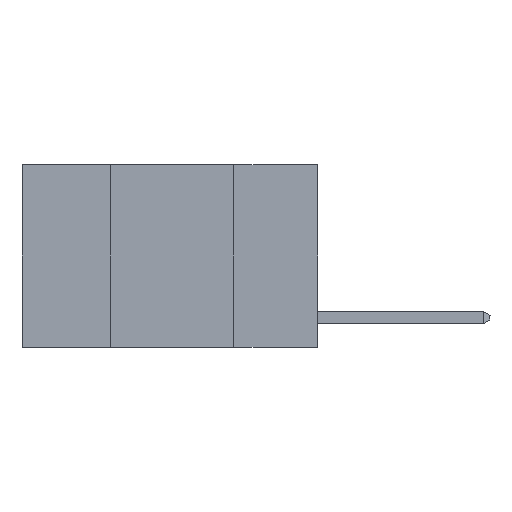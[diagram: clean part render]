
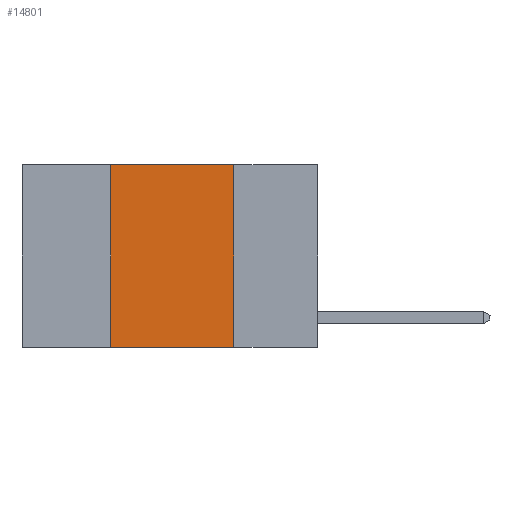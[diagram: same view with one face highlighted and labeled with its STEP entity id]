
A CAD part, left-side view. The second image highlights one B-rep face of the part: STEP entity #14801.
In plain terms, the highlighted planar face has unit normal (-1, 0, 0).
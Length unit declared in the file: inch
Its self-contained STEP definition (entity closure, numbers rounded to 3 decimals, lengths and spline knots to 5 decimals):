
#574 = LINE ( 'NONE', #12868, #12388 ) ;
#736 = CARTESIAN_POINT ( 'NONE',  ( 0., 0.6, -0.37 ) ) ;
#1305 = VECTOR ( 'NONE', #12393, 39.37008 ) ;
#1603 = DIRECTION ( 'NONE',  ( 0., 0., -1. ) ) ;
#1980 = ORIENTED_EDGE ( 'NONE', *, *, #10790, .F. ) ;
#2165 = LINE ( 'NONE', #2443, #1305 ) ;
#2443 = CARTESIAN_POINT ( 'NONE',  ( 0., 0.42, 0. ) ) ;
#3806 = AXIS2_PLACEMENT_3D ( 'NONE', #13803, #9630, #6894 ) ;
#4304 = VECTOR ( 'NONE', #1603, 39.37008 ) ;
#4466 = VERTEX_POINT ( 'NONE', #10080 ) ;
#4606 = ORIENTED_EDGE ( 'NONE', *, *, #11789, .F. ) ;
#4625 = CARTESIAN_POINT ( 'NONE',  ( 0., 0.17, -0.37 ) ) ;
#5789 = LINE ( 'NONE', #11376, #4304 ) ;
#6416 = DIRECTION ( 'NONE',  ( 0., -1., 0. ) ) ;
#6457 = ORIENTED_EDGE ( 'NONE', *, *, #16853, .F. ) ;
#6894 = DIRECTION ( 'NONE',  ( 0., 0., -1. ) ) ;
#7285 = CARTESIAN_POINT ( 'NONE',  ( 0., 0.42, 0. ) ) ;
#7732 = EDGE_CURVE ( 'NONE', #11258, #9309, #13419, .T. ) ;
#8183 = FACE_OUTER_BOUND ( 'NONE', #13230, .T. ) ;
#9309 = VERTEX_POINT ( 'NONE', #4625 ) ;
#9630 = DIRECTION ( 'NONE',  ( 1., 0., 0. ) ) ;
#10080 = CARTESIAN_POINT ( 'NONE',  ( 0., 0.17, 0. ) ) ;
#10790 = EDGE_CURVE ( 'NONE', #4466, #9309, #5789, .T. ) ;
#11258 = VERTEX_POINT ( 'NONE', #16481 ) ;
#11376 = CARTESIAN_POINT ( 'NONE',  ( 0., 0.17, 0. ) ) ;
#11789 = EDGE_CURVE ( 'NONE', #11258, #16188, #2165, .T. ) ;
#11837 = DIRECTION ( 'NONE',  ( 0., -1., 0. ) ) ;
#12309 = PLANE ( 'NONE',  #3806 ) ;
#12388 = VECTOR ( 'NONE', #11837, 39.37008 ) ;
#12393 = DIRECTION ( 'NONE',  ( 0., 0., 1. ) ) ;
#12868 = CARTESIAN_POINT ( 'NONE',  ( 0., 0.6, 0. ) ) ;
#13230 = EDGE_LOOP ( 'NONE', ( #1980, #6457, #4606, #15104 ) ) ;
#13419 = LINE ( 'NONE', #736, #15178 ) ;
#13803 = CARTESIAN_POINT ( 'NONE',  ( 0., 0.6, 0. ) ) ;
#14801 = ADVANCED_FACE ( 'NONE', ( #8183 ), #12309, .F. ) ;
#15104 = ORIENTED_EDGE ( 'NONE', *, *, #7732, .T. ) ;
#15178 = VECTOR ( 'NONE', #6416, 39.37008 ) ;
#16188 = VERTEX_POINT ( 'NONE', #7285 ) ;
#16481 = CARTESIAN_POINT ( 'NONE',  ( 0., 0.42, -0.37 ) ) ;
#16853 = EDGE_CURVE ( 'NONE', #16188, #4466, #574, .T. ) ;
